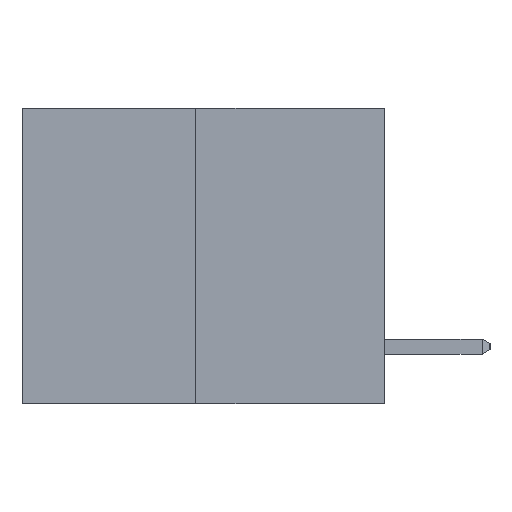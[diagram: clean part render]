
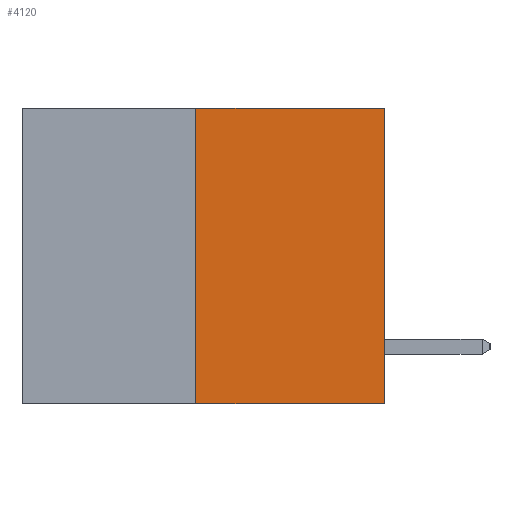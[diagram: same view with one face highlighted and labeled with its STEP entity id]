
A CAD part, left-side view. The second image highlights one B-rep face of the part: STEP entity #4120.
In plain terms, the highlighted planar face has unit normal (-1, 0, 0).
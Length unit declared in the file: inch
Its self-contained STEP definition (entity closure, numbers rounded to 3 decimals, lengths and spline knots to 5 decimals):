
#6 = LINE ( 'NONE', #23204, #2412 ) ;
#498 = CARTESIAN_POINT ( 'NONE',  ( 0., 0.6, 0. ) ) ;
#1506 = CARTESIAN_POINT ( 'NONE',  ( 0., 0.312, -0.49 ) ) ;
#2412 = VECTOR ( 'NONE', #26470, 39.37008 ) ;
#4120 = ADVANCED_FACE ( 'NONE', ( #8407 ), #11584, .F. ) ;
#4835 = EDGE_LOOP ( 'NONE', ( #12236, #20061, #5714, #22245 ) ) ;
#5714 = ORIENTED_EDGE ( 'NONE', *, *, #25018, .T. ) ;
#6079 = VECTOR ( 'NONE', #6271, 39.37008 ) ;
#6271 = DIRECTION ( 'NONE',  ( 0., 0., 1. ) ) ;
#7214 = CARTESIAN_POINT ( 'NONE',  ( 0., 0., 0. ) ) ;
#7469 = VECTOR ( 'NONE', #9237, 39.37008 ) ;
#8340 = VECTOR ( 'NONE', #27115, 39.37008 ) ;
#8407 = FACE_OUTER_BOUND ( 'NONE', #4835, .T. ) ;
#9237 = DIRECTION ( 'NONE',  ( 0., 0., 1. ) ) ;
#9458 = CARTESIAN_POINT ( 'NONE',  ( 0., 0., -0.49 ) ) ;
#9461 = CARTESIAN_POINT ( 'NONE',  ( 0., 0.6, -0.49 ) ) ;
#11584 = PLANE ( 'NONE',  #22641 ) ;
#12236 = ORIENTED_EDGE ( 'NONE', *, *, #16254, .F. ) ;
#13783 = DIRECTION ( 'NONE',  ( 1., 0., 0. ) ) ;
#15738 = EDGE_CURVE ( 'NONE', #22066, #25067, #6, .T. ) ;
#16179 = LINE ( 'NONE', #9461, #8340 ) ;
#16254 = EDGE_CURVE ( 'NONE', #22302, #22066, #27042, .T. ) ;
#19317 = CARTESIAN_POINT ( 'NONE',  ( 0., 0., 0. ) ) ;
#20061 = ORIENTED_EDGE ( 'NONE', *, *, #26827, .T. ) ;
#21775 = LINE ( 'NONE', #19317, #6079 ) ;
#22066 = VERTEX_POINT ( 'NONE', #23976 ) ;
#22245 = ORIENTED_EDGE ( 'NONE', *, *, #15738, .F. ) ;
#22302 = VERTEX_POINT ( 'NONE', #1506 ) ;
#22641 = AXIS2_PLACEMENT_3D ( 'NONE', #498, #13783, #24591 ) ;
#23204 = CARTESIAN_POINT ( 'NONE',  ( 0., 0.6, 0. ) ) ;
#23976 = CARTESIAN_POINT ( 'NONE',  ( 0., 0.312, 0. ) ) ;
#24417 = CARTESIAN_POINT ( 'NONE',  ( 0., 0.312, -0.49 ) ) ;
#24591 = DIRECTION ( 'NONE',  ( 0., 0., -1. ) ) ;
#24670 = VERTEX_POINT ( 'NONE', #9458 ) ;
#25018 = EDGE_CURVE ( 'NONE', #24670, #25067, #21775, .T. ) ;
#25067 = VERTEX_POINT ( 'NONE', #7214 ) ;
#26470 = DIRECTION ( 'NONE',  ( 0., -1., 0. ) ) ;
#26827 = EDGE_CURVE ( 'NONE', #22302, #24670, #16179, .T. ) ;
#27042 = LINE ( 'NONE', #24417, #7469 ) ;
#27115 = DIRECTION ( 'NONE',  ( 0., -1., 0. ) ) ;
